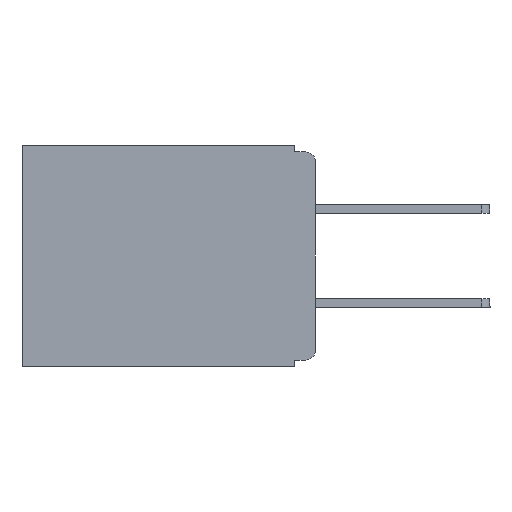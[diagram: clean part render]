
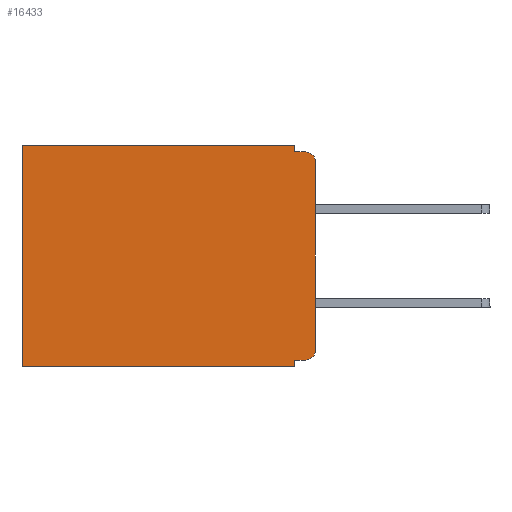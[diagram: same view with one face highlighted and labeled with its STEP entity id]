
A CAD part, left-side view. The second image highlights one B-rep face of the part: STEP entity #16433.
In plain terms, the highlighted planar face has unit normal (-1, 0, 0).
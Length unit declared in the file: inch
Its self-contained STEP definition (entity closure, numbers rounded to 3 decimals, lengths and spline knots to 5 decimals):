
#83 = DIRECTION ( 'NONE',  ( 0., 0., -1. ) ) ;
#131 = CARTESIAN_POINT ( 'NONE',  ( 0.3, 0., -0.01 ) ) ;
#264 = DIRECTION ( 'NONE',  ( 0., 0., -1. ) ) ;
#1101 = CARTESIAN_POINT ( 'NONE',  ( 0.3, 0., -0.33 ) ) ;
#1243 = CARTESIAN_POINT ( 'NONE',  ( 0.3, 0.015, -0.025 ) ) ;
#1261 = DIRECTION ( 'NONE',  ( -1., 0., 0. ) ) ;
#1269 = AXIS2_PLACEMENT_3D ( 'NONE', #1243, #1261, #1439 ) ;
#1439 = DIRECTION ( 'NONE',  ( 0., 0., -1. ) ) ;
#1488 = VERTEX_POINT ( 'NONE', #13205 ) ;
#1583 = VERTEX_POINT ( 'NONE', #15400 ) ;
#1835 = CARTESIAN_POINT ( 'NONE',  ( 0.3, 0., -0.33 ) ) ;
#2045 = CIRCLE ( 'NONE', #7674, 0.015 ) ;
#2127 = EDGE_CURVE ( 'NONE', #3130, #9106, #13966, .T. ) ;
#2350 = ORIENTED_EDGE ( 'NONE', *, *, #2127, .F. ) ;
#2487 = EDGE_CURVE ( 'NONE', #1488, #11419, #11778, .T. ) ;
#2665 = ORIENTED_EDGE ( 'NONE', *, *, #12572, .T. ) ;
#3074 = EDGE_CURVE ( 'NONE', #1488, #4447, #10524, .T. ) ;
#3130 = VERTEX_POINT ( 'NONE', #7775 ) ;
#3203 = VERTEX_POINT ( 'NONE', #3239 ) ;
#3239 = CARTESIAN_POINT ( 'NONE',  ( 0.3, 0.031, -0.32 ) ) ;
#3389 = VECTOR ( 'NONE', #3757, 39.37008 ) ;
#3408 = VERTEX_POINT ( 'NONE', #11084 ) ;
#3451 = EDGE_CURVE ( 'NONE', #3408, #4447, #2045, .T. ) ;
#3757 = DIRECTION ( 'NONE',  ( 0., 1., 0. ) ) ;
#3921 = EDGE_CURVE ( 'NONE', #7420, #11419, #16104, .T. ) ;
#4447 = VERTEX_POINT ( 'NONE', #9783 ) ;
#4780 = CARTESIAN_POINT ( 'NONE',  ( 0.3, 0., -0.33 ) ) ;
#5411 = EDGE_CURVE ( 'NONE', #3203, #3130, #10276, .T. ) ;
#5933 = LINE ( 'NONE', #10716, #16665 ) ;
#5940 = EDGE_LOOP ( 'NONE', ( #16915, #11514, #11327, #8556, #10449, #2665, #2350, #8054, #7769, #16407 ) ) ;
#6158 = DIRECTION ( 'NONE',  ( 0., 0., -1. ) ) ;
#6554 = DIRECTION ( 'NONE',  ( 0., 0., -1. ) ) ;
#6731 = VECTOR ( 'NONE', #6756, 39.37008 ) ;
#6756 = DIRECTION ( 'NONE',  ( 0., 0., -1. ) ) ;
#6840 = CARTESIAN_POINT ( 'NONE',  ( 0.3, 0.015, -0.305 ) ) ;
#6859 = DIRECTION ( 'NONE',  ( 0., -1., 0. ) ) ;
#6971 = CARTESIAN_POINT ( 'NONE',  ( 0.3, 0.031, -0.01 ) ) ;
#7009 = VECTOR ( 'NONE', #6554, 39.37008 ) ;
#7420 = VERTEX_POINT ( 'NONE', #6971 ) ;
#7572 = EDGE_CURVE ( 'NONE', #3408, #3203, #5933, .T. ) ;
#7674 = AXIS2_PLACEMENT_3D ( 'NONE', #6840, #7826, #14820 ) ;
#7769 = ORIENTED_EDGE ( 'NONE', *, *, #7572, .F. ) ;
#7775 = CARTESIAN_POINT ( 'NONE',  ( 0.3, 0.031, -0.33 ) ) ;
#7826 = DIRECTION ( 'NONE',  ( -1., 0., 0. ) ) ;
#8054 = ORIENTED_EDGE ( 'NONE', *, *, #5411, .F. ) ;
#8111 = VECTOR ( 'NONE', #83, 39.37008 ) ;
#8475 = CARTESIAN_POINT ( 'NONE',  ( 0.3, 0.015, -0.01 ) ) ;
#8556 = ORIENTED_EDGE ( 'NONE', *, *, #15746, .F. ) ;
#9049 = CARTESIAN_POINT ( 'NONE',  ( 0.3, 0.031, 0. ) ) ;
#9080 = CARTESIAN_POINT ( 'NONE',  ( 0.3, 0.031, -0.33 ) ) ;
#9106 = VERTEX_POINT ( 'NONE', #10603 ) ;
#9177 = CARTESIAN_POINT ( 'NONE',  ( 0.3, 0., 0. ) ) ;
#9783 = CARTESIAN_POINT ( 'NONE',  ( 0.3, 0., -0.305 ) ) ;
#10080 = LINE ( 'NONE', #15040, #10878 ) ;
#10276 = LINE ( 'NONE', #9080, #6731 ) ;
#10449 = ORIENTED_EDGE ( 'NONE', *, *, #13441, .T. ) ;
#10524 = LINE ( 'NONE', #1835, #7009 ) ;
#10603 = CARTESIAN_POINT ( 'NONE',  ( 0.3, 0.437, -0.33 ) ) ;
#10716 = CARTESIAN_POINT ( 'NONE',  ( 0.3, 0., -0.32 ) ) ;
#10878 = VECTOR ( 'NONE', #264, 39.37008 ) ;
#11084 = CARTESIAN_POINT ( 'NONE',  ( 0.3, 0.015, -0.32 ) ) ;
#11327 = ORIENTED_EDGE ( 'NONE', *, *, #3921, .F. ) ;
#11419 = VERTEX_POINT ( 'NONE', #8475 ) ;
#11449 = PLANE ( 'NONE',  #13585 ) ;
#11514 = ORIENTED_EDGE ( 'NONE', *, *, #2487, .T. ) ;
#11602 = LINE ( 'NONE', #12259, #8111 ) ;
#11671 = VERTEX_POINT ( 'NONE', #9049 ) ;
#11778 = CIRCLE ( 'NONE', #1269, 0.015 ) ;
#12259 = CARTESIAN_POINT ( 'NONE',  ( 0.3, 0.437, -0.33 ) ) ;
#12398 = VECTOR ( 'NONE', #16775, 39.37008 ) ;
#12572 = EDGE_CURVE ( 'NONE', #1583, #9106, #11602, .T. ) ;
#12766 = VECTOR ( 'NONE', #6859, 39.37008 ) ;
#13205 = CARTESIAN_POINT ( 'NONE',  ( 0.3, 0., -0.025 ) ) ;
#13441 = EDGE_CURVE ( 'NONE', #11671, #1583, #15773, .T. ) ;
#13585 = AXIS2_PLACEMENT_3D ( 'NONE', #4780, #13997, #6158 ) ;
#13966 = LINE ( 'NONE', #1101, #3389 ) ;
#13997 = DIRECTION ( 'NONE',  ( 1., 0., 0. ) ) ;
#14820 = DIRECTION ( 'NONE',  ( 0., 0., -1. ) ) ;
#15040 = CARTESIAN_POINT ( 'NONE',  ( 0.3, 0.031, 0. ) ) ;
#15400 = CARTESIAN_POINT ( 'NONE',  ( 0.3, 0.437, 0. ) ) ;
#15458 = FACE_OUTER_BOUND ( 'NONE', #5940, .T. ) ;
#15746 = EDGE_CURVE ( 'NONE', #11671, #7420, #10080, .T. ) ;
#15773 = LINE ( 'NONE', #9177, #12398 ) ;
#16104 = LINE ( 'NONE', #131, #12766 ) ;
#16407 = ORIENTED_EDGE ( 'NONE', *, *, #3451, .T. ) ;
#16433 = ADVANCED_FACE ( 'NONE', ( #15458 ), #11449, .F. ) ;
#16665 = VECTOR ( 'NONE', #16741, 39.37008 ) ;
#16741 = DIRECTION ( 'NONE',  ( 0., 1., 0. ) ) ;
#16775 = DIRECTION ( 'NONE',  ( 0., 1., 0. ) ) ;
#16915 = ORIENTED_EDGE ( 'NONE', *, *, #3074, .F. ) ;
